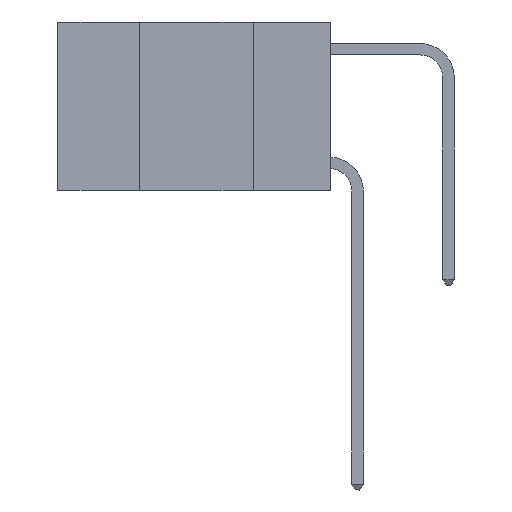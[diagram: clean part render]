
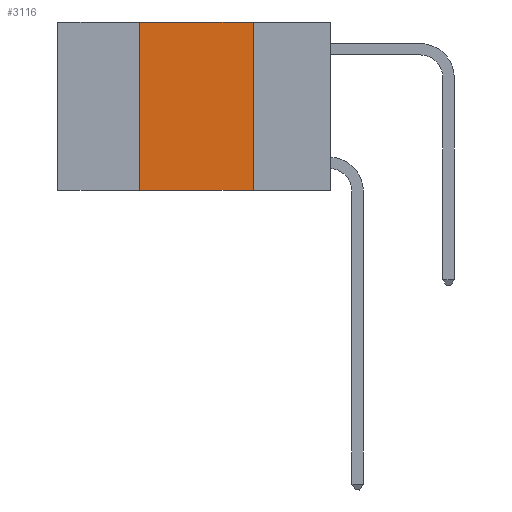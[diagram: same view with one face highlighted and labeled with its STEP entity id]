
A CAD part, left-side view. The second image highlights one B-rep face of the part: STEP entity #3116.
In plain terms, the highlighted planar face has unit normal (-1, 0, 0).
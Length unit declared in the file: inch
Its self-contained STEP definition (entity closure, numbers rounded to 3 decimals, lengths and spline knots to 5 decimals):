
#811 = LINE ( 'NONE', #1359, #15515 ) ;
#1359 = CARTESIAN_POINT ( 'NONE',  ( 0., 0.6, -0.37 ) ) ;
#1708 = CARTESIAN_POINT ( 'NONE',  ( 0., 0.17, 0. ) ) ;
#2220 = CARTESIAN_POINT ( 'NONE',  ( 0., 0.17, -0.37 ) ) ;
#2728 = DIRECTION ( 'NONE',  ( 1., 0., 0. ) ) ;
#2937 = VERTEX_POINT ( 'NONE', #18174 ) ;
#3116 = ADVANCED_FACE ( 'NONE', ( #5345 ), #4959, .F. ) ;
#3496 = VERTEX_POINT ( 'NONE', #15609 ) ;
#3684 = ORIENTED_EDGE ( 'NONE', *, *, #11279, .F. ) ;
#4943 = EDGE_CURVE ( 'NONE', #3496, #15355, #811, .T. ) ;
#4959 = PLANE ( 'NONE',  #16069 ) ;
#5345 = FACE_OUTER_BOUND ( 'NONE', #15468, .T. ) ;
#6776 = DIRECTION ( 'NONE',  ( 0., -1., 0. ) ) ;
#6986 = ORIENTED_EDGE ( 'NONE', *, *, #17600, .F. ) ;
#8103 = VECTOR ( 'NONE', #14552, 39.37008 ) ;
#8611 = VECTOR ( 'NONE', #9181, 39.37008 ) ;
#9181 = DIRECTION ( 'NONE',  ( 0., 0., 1. ) ) ;
#10871 = EDGE_CURVE ( 'NONE', #2937, #12224, #14893, .T. ) ;
#11045 = CARTESIAN_POINT ( 'NONE',  ( 0., 0.6, 0. ) ) ;
#11279 = EDGE_CURVE ( 'NONE', #3496, #2937, #15754, .T. ) ;
#11694 = ORIENTED_EDGE ( 'NONE', *, *, #4943, .T. ) ;
#11926 = LINE ( 'NONE', #1708, #8103 ) ;
#12091 = CARTESIAN_POINT ( 'NONE',  ( 0., 0.6, 0. ) ) ;
#12224 = VERTEX_POINT ( 'NONE', #18368 ) ;
#12274 = DIRECTION ( 'NONE',  ( 0., 0., -1. ) ) ;
#13511 = CARTESIAN_POINT ( 'NONE',  ( 0., 0.42, 0. ) ) ;
#14552 = DIRECTION ( 'NONE',  ( 0., 0., -1. ) ) ;
#14893 = LINE ( 'NONE', #11045, #17774 ) ;
#15355 = VERTEX_POINT ( 'NONE', #2220 ) ;
#15468 = EDGE_LOOP ( 'NONE', ( #6986, #18348, #3684, #11694 ) ) ;
#15515 = VECTOR ( 'NONE', #17066, 39.37008 ) ;
#15609 = CARTESIAN_POINT ( 'NONE',  ( 0., 0.42, -0.37 ) ) ;
#15754 = LINE ( 'NONE', #13511, #8611 ) ;
#16069 = AXIS2_PLACEMENT_3D ( 'NONE', #12091, #2728, #12274 ) ;
#17066 = DIRECTION ( 'NONE',  ( 0., -1., 0. ) ) ;
#17600 = EDGE_CURVE ( 'NONE', #12224, #15355, #11926, .T. ) ;
#17774 = VECTOR ( 'NONE', #6776, 39.37008 ) ;
#18174 = CARTESIAN_POINT ( 'NONE',  ( 0., 0.42, 0. ) ) ;
#18348 = ORIENTED_EDGE ( 'NONE', *, *, #10871, .F. ) ;
#18368 = CARTESIAN_POINT ( 'NONE',  ( 0., 0.17, 0. ) ) ;
